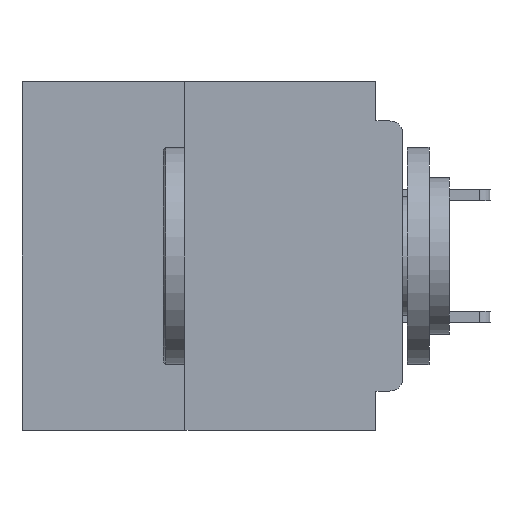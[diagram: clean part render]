
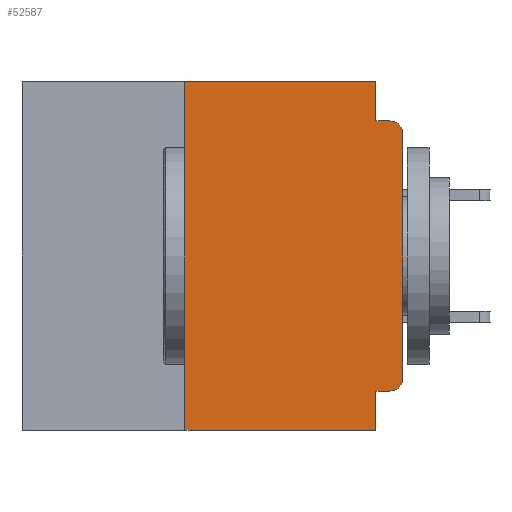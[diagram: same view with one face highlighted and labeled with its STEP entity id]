
A CAD part, left-side view. The second image highlights one B-rep face of the part: STEP entity #52587.
In plain terms, the highlighted planar face has unit normal (-1, 0, 0).
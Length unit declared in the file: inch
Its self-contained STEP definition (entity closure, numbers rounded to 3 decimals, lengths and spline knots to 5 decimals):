
#736 = VECTOR ( 'NONE', #25979, 39.37008 ) ;
#831 = DIRECTION ( 'NONE',  ( 0., 0., -1. ) ) ;
#1085 = VERTEX_POINT ( 'NONE', #60331 ) ;
#1869 = LINE ( 'NONE', #38731, #50984 ) ;
#2020 = CARTESIAN_POINT ( 'NONE',  ( 0., 0.437, 0. ) ) ;
#2280 = ORIENTED_EDGE ( 'NONE', *, *, #7282, .T. ) ;
#2486 = DIRECTION ( 'NONE',  ( 0., 0., -1. ) ) ;
#4519 = VERTEX_POINT ( 'NONE', #36807 ) ;
#4528 = CARTESIAN_POINT ( 'NONE',  ( 0., 0.25, -0.4 ) ) ;
#4986 = EDGE_CURVE ( 'NONE', #1085, #4519, #49853, .T. ) ;
#5289 = CARTESIAN_POINT ( 'NONE',  ( 0., 0.015, -0.06 ) ) ;
#5876 = VECTOR ( 'NONE', #23043, 39.37008 ) ;
#6370 = EDGE_CURVE ( 'NONE', #57739, #19770, #12655, .T. ) ;
#7282 = EDGE_CURVE ( 'NONE', #19289, #58729, #18651, .T. ) ;
#7633 = CARTESIAN_POINT ( 'NONE',  ( 0., 0.25, 0. ) ) ;
#8868 = VERTEX_POINT ( 'NONE', #27840 ) ;
#10116 = DIRECTION ( 'NONE',  ( 0., 0., -1. ) ) ;
#10524 = CIRCLE ( 'NONE', #35642, 0.015 ) ;
#11423 = CARTESIAN_POINT ( 'NONE',  ( 0., 0., -0.355 ) ) ;
#12299 = ORIENTED_EDGE ( 'NONE', *, *, #33177, .F. ) ;
#12655 = LINE ( 'NONE', #44714, #20902 ) ;
#13233 = VERTEX_POINT ( 'NONE', #37664 ) ;
#13981 = DIRECTION ( 'NONE',  ( 0., -1., 0. ) ) ;
#16241 = DIRECTION ( 'NONE',  ( 0., 1., 0. ) ) ;
#16957 = CARTESIAN_POINT ( 'NONE',  ( 0., 0.031, 0. ) ) ;
#17595 = EDGE_CURVE ( 'NONE', #19289, #57739, #46154, .T. ) ;
#18191 = VECTOR ( 'NONE', #2486, 39.37008 ) ;
#18389 = DIRECTION ( 'NONE',  ( -1., 0., 0. ) ) ;
#18651 = LINE ( 'NONE', #37128, #5876 ) ;
#19289 = VERTEX_POINT ( 'NONE', #46402 ) ;
#19770 = VERTEX_POINT ( 'NONE', #35780 ) ;
#19799 = AXIS2_PLACEMENT_3D ( 'NONE', #46781, #18389, #51537 ) ;
#20902 = VECTOR ( 'NONE', #21073, 39.37008 ) ;
#21073 = DIRECTION ( 'NONE',  ( 0., -1., 0. ) ) ;
#21222 = CARTESIAN_POINT ( 'NONE',  ( 0., 0., 0. ) ) ;
#23043 = DIRECTION ( 'NONE',  ( 0., -1., 0. ) ) ;
#24114 = LINE ( 'NONE', #11423, #58963 ) ;
#24989 = ORIENTED_EDGE ( 'NONE', *, *, #47083, .F. ) ;
#25299 = ORIENTED_EDGE ( 'NONE', *, *, #54089, .T. ) ;
#25682 = AXIS2_PLACEMENT_3D ( 'NONE', #2020, #26007, #59179 ) ;
#25979 = DIRECTION ( 'NONE',  ( 0., 0., 1. ) ) ;
#26007 = DIRECTION ( 'NONE',  ( 1., 0., 0. ) ) ;
#27775 = EDGE_CURVE ( 'NONE', #19770, #8868, #43390, .T. ) ;
#27840 = CARTESIAN_POINT ( 'NONE',  ( 0., 0.031, -0.045 ) ) ;
#28395 = ORIENTED_EDGE ( 'NONE', *, *, #27775, .F. ) ;
#28781 = EDGE_CURVE ( 'NONE', #4519, #54742, #10524, .T. ) ;
#29335 = ORIENTED_EDGE ( 'NONE', *, *, #4986, .T. ) ;
#33177 = EDGE_CURVE ( 'NONE', #13233, #58729, #1869, .T. ) ;
#33489 = CARTESIAN_POINT ( 'NONE',  ( 0., 0.015, -0.045 ) ) ;
#35372 = PLANE ( 'NONE',  #25682 ) ;
#35642 = AXIS2_PLACEMENT_3D ( 'NONE', #5289, #38616, #10116 ) ;
#35780 = CARTESIAN_POINT ( 'NONE',  ( 0., 0.031, 0. ) ) ;
#36807 = CARTESIAN_POINT ( 'NONE',  ( 0., 0., -0.06 ) ) ;
#37128 = CARTESIAN_POINT ( 'NONE',  ( 0., 0.437, -0.4 ) ) ;
#37336 = CARTESIAN_POINT ( 'NONE',  ( 0., 0.031, -0.4 ) ) ;
#37383 = ORIENTED_EDGE ( 'NONE', *, *, #17595, .F. ) ;
#37664 = CARTESIAN_POINT ( 'NONE',  ( 0., 0.031, -0.355 ) ) ;
#38080 = ORIENTED_EDGE ( 'NONE', *, *, #59706, .F. ) ;
#38281 = VECTOR ( 'NONE', #13981, 39.37008 ) ;
#38616 = DIRECTION ( 'NONE',  ( -1., 0., 0. ) ) ;
#38731 = CARTESIAN_POINT ( 'NONE',  ( 0., 0.031, -0.4 ) ) ;
#39775 = FACE_OUTER_BOUND ( 'NONE', #50301, .T. ) ;
#42437 = CARTESIAN_POINT ( 'NONE',  ( 0., 0., -0.045 ) ) ;
#43261 = CIRCLE ( 'NONE', #19799, 0.015 ) ;
#43390 = LINE ( 'NONE', #16957, #18191 ) ;
#44714 = CARTESIAN_POINT ( 'NONE',  ( 0., 0.437, 0. ) ) ;
#45529 = VERTEX_POINT ( 'NONE', #58249 ) ;
#46154 = LINE ( 'NONE', #4528, #57284 ) ;
#46402 = CARTESIAN_POINT ( 'NONE',  ( 0., 0.25, -0.4 ) ) ;
#46781 = CARTESIAN_POINT ( 'NONE',  ( 0., 0.015, -0.34 ) ) ;
#47083 = EDGE_CURVE ( 'NONE', #8868, #54742, #50879, .T. ) ;
#49853 = LINE ( 'NONE', #21222, #736 ) ;
#50301 = EDGE_LOOP ( 'NONE', ( #29335, #58964, #24989, #28395, #57980, #37383, #2280, #12299, #38080, #25299 ) ) ;
#50879 = LINE ( 'NONE', #42437, #38281 ) ;
#50984 = VECTOR ( 'NONE', #831, 39.37008 ) ;
#51537 = DIRECTION ( 'NONE',  ( 0., 0., -1. ) ) ;
#52587 = ADVANCED_FACE ( 'NONE', ( #39775 ), #35372, .F. ) ;
#54089 = EDGE_CURVE ( 'NONE', #45529, #1085, #43261, .T. ) ;
#54742 = VERTEX_POINT ( 'NONE', #33489 ) ;
#56725 = DIRECTION ( 'NONE',  ( 0., 0., 1. ) ) ;
#57284 = VECTOR ( 'NONE', #56725, 39.37008 ) ;
#57739 = VERTEX_POINT ( 'NONE', #7633 ) ;
#57980 = ORIENTED_EDGE ( 'NONE', *, *, #6370, .F. ) ;
#58249 = CARTESIAN_POINT ( 'NONE',  ( 0., 0.015, -0.355 ) ) ;
#58729 = VERTEX_POINT ( 'NONE', #37336 ) ;
#58963 = VECTOR ( 'NONE', #16241, 39.37008 ) ;
#58964 = ORIENTED_EDGE ( 'NONE', *, *, #28781, .T. ) ;
#59179 = DIRECTION ( 'NONE',  ( 0., 0., -1. ) ) ;
#59706 = EDGE_CURVE ( 'NONE', #45529, #13233, #24114, .T. ) ;
#60331 = CARTESIAN_POINT ( 'NONE',  ( 0., 0., -0.34 ) ) ;
